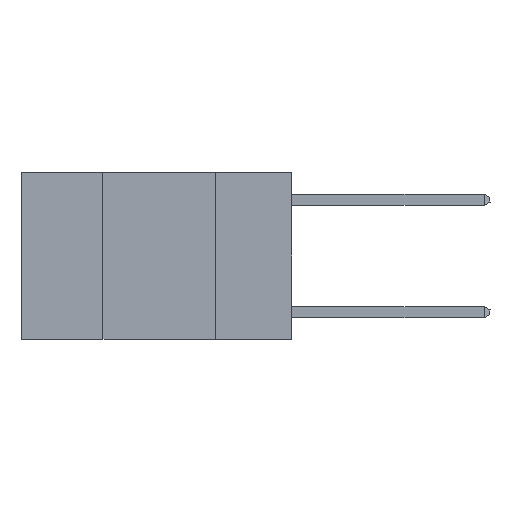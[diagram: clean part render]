
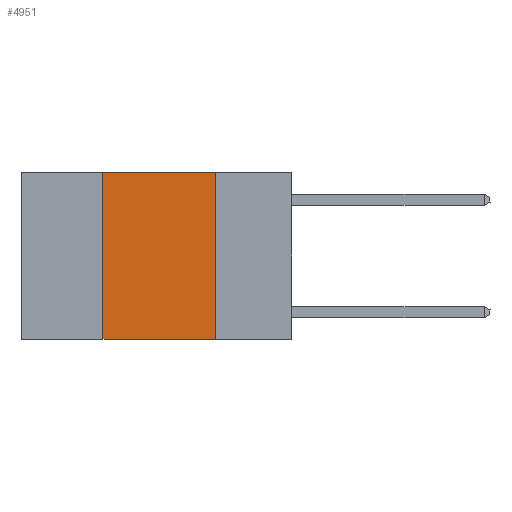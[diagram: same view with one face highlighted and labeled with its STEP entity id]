
A CAD part, left-side view. The second image highlights one B-rep face of the part: STEP entity #4951.
In plain terms, the highlighted planar face has unit normal (-1, 0, 0).
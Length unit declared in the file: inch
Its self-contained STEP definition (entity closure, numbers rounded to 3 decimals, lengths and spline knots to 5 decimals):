
#63 = DIRECTION ( 'NONE',  ( 0., 0., -1. ) ) ;
#447 = VERTEX_POINT ( 'NONE', #3925 ) ;
#544 = ORIENTED_EDGE ( 'NONE', *, *, #1628, .F. ) ;
#1076 = AXIS2_PLACEMENT_3D ( 'NONE', #4168, #8640, #1632 ) ;
#1628 = EDGE_CURVE ( 'NONE', #4577, #8326, #6583, .T. ) ;
#1632 = DIRECTION ( 'NONE',  ( 0., 0., -1. ) ) ;
#2396 = ORIENTED_EDGE ( 'NONE', *, *, #11194, .F. ) ;
#3196 = LINE ( 'NONE', #7407, #11727 ) ;
#3446 = EDGE_CURVE ( 'NONE', #8326, #3762, #12936, .T. ) ;
#3651 = VECTOR ( 'NONE', #8830, 39.37008 ) ;
#3762 = VERTEX_POINT ( 'NONE', #14466 ) ;
#3925 = CARTESIAN_POINT ( 'NONE',  ( 0., 0.42, -0.37 ) ) ;
#3963 = FACE_OUTER_BOUND ( 'NONE', #14249, .T. ) ;
#4168 = CARTESIAN_POINT ( 'NONE',  ( 0., 0.6, 0. ) ) ;
#4577 = VERTEX_POINT ( 'NONE', #7648 ) ;
#4951 = ADVANCED_FACE ( 'NONE', ( #3963 ), #7585, .F. ) ;
#6583 = LINE ( 'NONE', #9908, #11964 ) ;
#7407 = CARTESIAN_POINT ( 'NONE',  ( 0., 0.42, 0. ) ) ;
#7585 = PLANE ( 'NONE',  #1076 ) ;
#7648 = CARTESIAN_POINT ( 'NONE',  ( 0., 0.42, 0. ) ) ;
#7768 = CARTESIAN_POINT ( 'NONE',  ( 0., 0.6, -0.37 ) ) ;
#8326 = VERTEX_POINT ( 'NONE', #10078 ) ;
#8466 = DIRECTION ( 'NONE',  ( 0., 0., 1. ) ) ;
#8640 = DIRECTION ( 'NONE',  ( 1., 0., 0. ) ) ;
#8691 = VECTOR ( 'NONE', #63, 39.37008 ) ;
#8830 = DIRECTION ( 'NONE',  ( 0., -1., 0. ) ) ;
#8918 = ORIENTED_EDGE ( 'NONE', *, *, #9004, .T. ) ;
#9004 = EDGE_CURVE ( 'NONE', #447, #3762, #12463, .T. ) ;
#9908 = CARTESIAN_POINT ( 'NONE',  ( 0., 0.6, 0. ) ) ;
#10078 = CARTESIAN_POINT ( 'NONE',  ( 0., 0.17, 0. ) ) ;
#10811 = ORIENTED_EDGE ( 'NONE', *, *, #3446, .F. ) ;
#10846 = DIRECTION ( 'NONE',  ( 0., -1., 0. ) ) ;
#10881 = CARTESIAN_POINT ( 'NONE',  ( 0., 0.17, 0. ) ) ;
#11194 = EDGE_CURVE ( 'NONE', #447, #4577, #3196, .T. ) ;
#11727 = VECTOR ( 'NONE', #8466, 39.37008 ) ;
#11964 = VECTOR ( 'NONE', #10846, 39.37008 ) ;
#12463 = LINE ( 'NONE', #7768, #3651 ) ;
#12936 = LINE ( 'NONE', #10881, #8691 ) ;
#14249 = EDGE_LOOP ( 'NONE', ( #10811, #544, #2396, #8918 ) ) ;
#14466 = CARTESIAN_POINT ( 'NONE',  ( 0., 0.17, -0.37 ) ) ;
